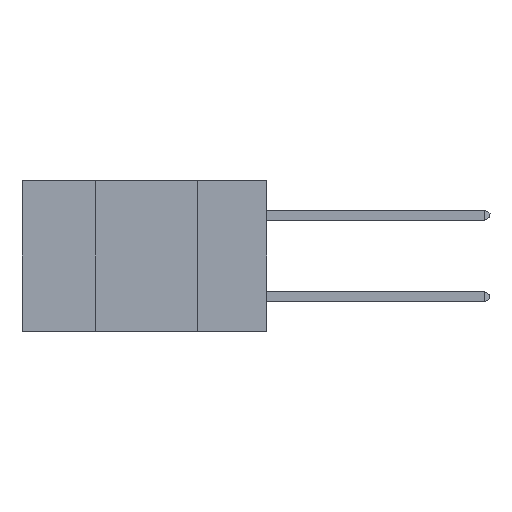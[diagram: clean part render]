
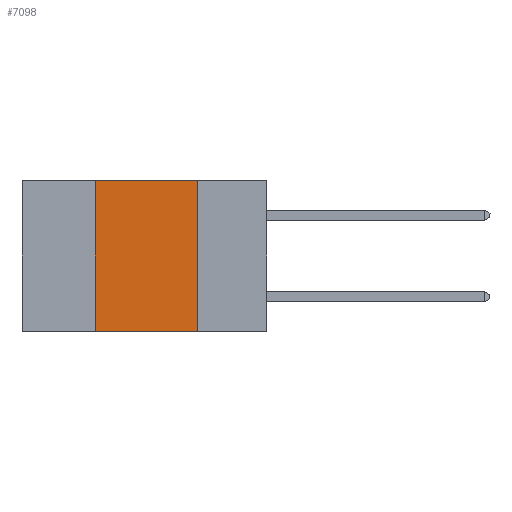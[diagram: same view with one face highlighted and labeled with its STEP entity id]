
A CAD part, left-side view. The second image highlights one B-rep face of the part: STEP entity #7098.
In plain terms, the highlighted planar face has unit normal (-1, 0, 0).
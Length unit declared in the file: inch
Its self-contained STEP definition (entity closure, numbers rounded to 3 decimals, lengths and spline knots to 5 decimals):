
#360 = VERTEX_POINT ( 'NONE', #6563 ) ;
#1034 = CARTESIAN_POINT ( 'NONE',  ( 0., 0.42, 0. ) ) ;
#1341 = EDGE_CURVE ( 'NONE', #14438, #11014, #2612, .T. ) ;
#2270 = EDGE_LOOP ( 'NONE', ( #5246, #5334, #5404, #5424 ) ) ;
#2308 = CARTESIAN_POINT ( 'NONE',  ( 0., 0.42, -0.37 ) ) ;
#2612 = LINE ( 'NONE', #10144, #5823 ) ;
#2990 = CARTESIAN_POINT ( 'NONE',  ( 0., 0.17, 0. ) ) ;
#3088 = DIRECTION ( 'NONE',  ( 0., -1., 0. ) ) ;
#5246 = ORIENTED_EDGE ( 'NONE', *, *, #5580, .F. ) ;
#5334 = ORIENTED_EDGE ( 'NONE', *, *, #1341, .F. ) ;
#5404 = ORIENTED_EDGE ( 'NONE', *, *, #6358, .F. ) ;
#5424 = ORIENTED_EDGE ( 'NONE', *, *, #8703, .T. ) ;
#5580 = EDGE_CURVE ( 'NONE', #11014, #360, #7721, .T. ) ;
#5823 = VECTOR ( 'NONE', #10096, 39.37008 ) ;
#6054 = VECTOR ( 'NONE', #12407, 39.37008 ) ;
#6358 = EDGE_CURVE ( 'NONE', #12518, #14438, #12926, .T. ) ;
#6563 = CARTESIAN_POINT ( 'NONE',  ( 0., 0.17, -0.37 ) ) ;
#7098 = ADVANCED_FACE ( 'NONE', ( #9615 ), #13557, .F. ) ;
#7134 = CARTESIAN_POINT ( 'NONE',  ( 0., 0.6, 0. ) ) ;
#7476 = AXIS2_PLACEMENT_3D ( 'NONE', #7134, #14657, #8302 ) ;
#7721 = LINE ( 'NONE', #12185, #10643 ) ;
#8302 = DIRECTION ( 'NONE',  ( 0., 0., -1. ) ) ;
#8703 = EDGE_CURVE ( 'NONE', #12518, #360, #9810, .T. ) ;
#8965 = CARTESIAN_POINT ( 'NONE',  ( 0., 0.6, -0.37 ) ) ;
#9615 = FACE_OUTER_BOUND ( 'NONE', #2270, .T. ) ;
#9810 = LINE ( 'NONE', #8965, #10483 ) ;
#10096 = DIRECTION ( 'NONE',  ( 0., -1., 0. ) ) ;
#10144 = CARTESIAN_POINT ( 'NONE',  ( 0., 0.6, 0. ) ) ;
#10483 = VECTOR ( 'NONE', #3088, 39.37008 ) ;
#10643 = VECTOR ( 'NONE', #13239, 39.37008 ) ;
#11014 = VERTEX_POINT ( 'NONE', #2990 ) ;
#12185 = CARTESIAN_POINT ( 'NONE',  ( 0., 0.17, 0. ) ) ;
#12407 = DIRECTION ( 'NONE',  ( 0., 0., 1. ) ) ;
#12518 = VERTEX_POINT ( 'NONE', #2308 ) ;
#12926 = LINE ( 'NONE', #14460, #6054 ) ;
#13239 = DIRECTION ( 'NONE',  ( 0., 0., -1. ) ) ;
#13557 = PLANE ( 'NONE',  #7476 ) ;
#14438 = VERTEX_POINT ( 'NONE', #1034 ) ;
#14460 = CARTESIAN_POINT ( 'NONE',  ( 0., 0.42, 0. ) ) ;
#14657 = DIRECTION ( 'NONE',  ( 1., 0., 0. ) ) ;
